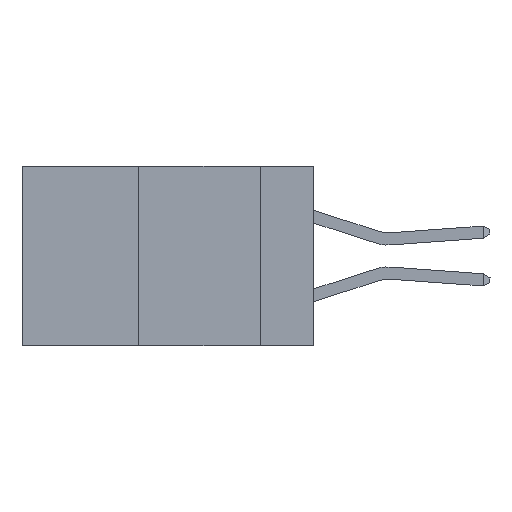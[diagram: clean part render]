
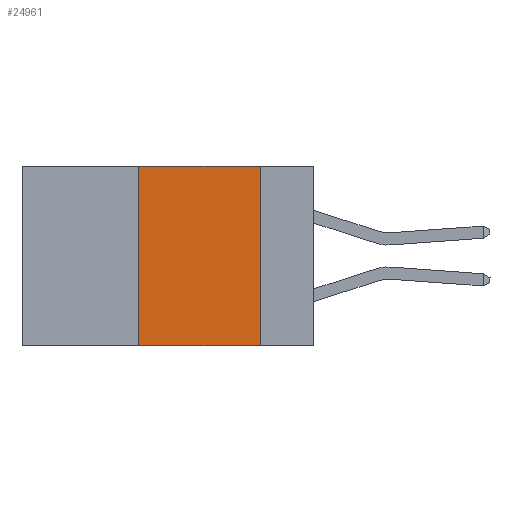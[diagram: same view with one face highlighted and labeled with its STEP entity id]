
A CAD part, left-side view. The second image highlights one B-rep face of the part: STEP entity #24961.
In plain terms, the highlighted planar face has unit normal (-1, 0, 0).
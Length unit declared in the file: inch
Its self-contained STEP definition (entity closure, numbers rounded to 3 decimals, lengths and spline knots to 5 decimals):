
#431 = DIRECTION ( 'NONE',  ( 0., -1., 0. ) ) ;
#435 = ORIENTED_EDGE ( 'NONE', *, *, #20167, .F. ) ;
#1150 = EDGE_CURVE ( 'NONE', #20917, #2444, #10535, .T. ) ;
#1480 = LINE ( 'NONE', #8966, #17590 ) ;
#1818 = AXIS2_PLACEMENT_3D ( 'NONE', #3328, #18026, #5453 ) ;
#2152 = VERTEX_POINT ( 'NONE', #5410 ) ;
#2354 = VERTEX_POINT ( 'NONE', #18714 ) ;
#2444 = VERTEX_POINT ( 'NONE', #8542 ) ;
#3328 = CARTESIAN_POINT ( 'NONE',  ( 0., 0.6, 0. ) ) ;
#4347 = EDGE_CURVE ( 'NONE', #20917, #2354, #13115, .T. ) ;
#5410 = CARTESIAN_POINT ( 'NONE',  ( 0., 0.11, 0. ) ) ;
#5453 = DIRECTION ( 'NONE',  ( 0., 0., -1. ) ) ;
#6529 = EDGE_LOOP ( 'NONE', ( #11014, #435, #6750, #17912 ) ) ;
#6750 = ORIENTED_EDGE ( 'NONE', *, *, #1150, .F. ) ;
#8542 = CARTESIAN_POINT ( 'NONE',  ( 0., 0.36, 0. ) ) ;
#8966 = CARTESIAN_POINT ( 'NONE',  ( 0., 0.6, 0. ) ) ;
#9725 = DIRECTION ( 'NONE',  ( 0., -1., 0. ) ) ;
#10535 = LINE ( 'NONE', #17285, #27228 ) ;
#10963 = EDGE_CURVE ( 'NONE', #2152, #2354, #18289, .T. ) ;
#11014 = ORIENTED_EDGE ( 'NONE', *, *, #10963, .F. ) ;
#13115 = LINE ( 'NONE', #15937, #18062 ) ;
#13308 = CARTESIAN_POINT ( 'NONE',  ( 0., 0.36, -0.37 ) ) ;
#13795 = PLANE ( 'NONE',  #1818 ) ;
#15704 = CARTESIAN_POINT ( 'NONE',  ( 0., 0.11, 0. ) ) ;
#15937 = CARTESIAN_POINT ( 'NONE',  ( 0., 0.6, -0.37 ) ) ;
#17285 = CARTESIAN_POINT ( 'NONE',  ( 0., 0.36, 0. ) ) ;
#17590 = VECTOR ( 'NONE', #431, 39.37008 ) ;
#17621 = VECTOR ( 'NONE', #17818, 39.37008 ) ;
#17818 = DIRECTION ( 'NONE',  ( 0., 0., -1. ) ) ;
#17912 = ORIENTED_EDGE ( 'NONE', *, *, #4347, .T. ) ;
#18026 = DIRECTION ( 'NONE',  ( 1., 0., 0. ) ) ;
#18062 = VECTOR ( 'NONE', #9725, 39.37008 ) ;
#18289 = LINE ( 'NONE', #15704, #17621 ) ;
#18714 = CARTESIAN_POINT ( 'NONE',  ( 0., 0.11, -0.37 ) ) ;
#20167 = EDGE_CURVE ( 'NONE', #2444, #2152, #1480, .T. ) ;
#20917 = VERTEX_POINT ( 'NONE', #13308 ) ;
#23498 = DIRECTION ( 'NONE',  ( 0., 0., 1. ) ) ;
#24783 = FACE_OUTER_BOUND ( 'NONE', #6529, .T. ) ;
#24961 = ADVANCED_FACE ( 'NONE', ( #24783 ), #13795, .F. ) ;
#27228 = VECTOR ( 'NONE', #23498, 39.37008 ) ;
